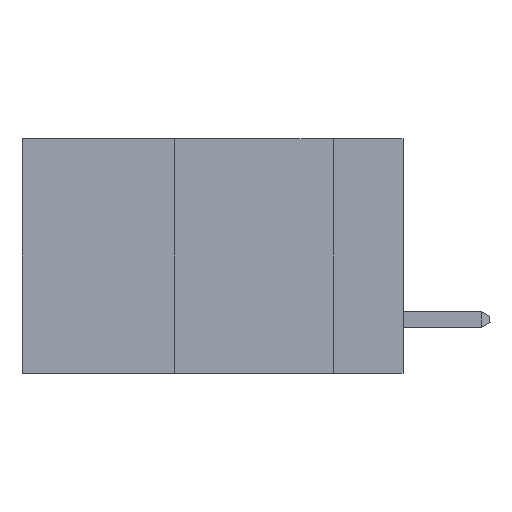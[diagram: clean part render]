
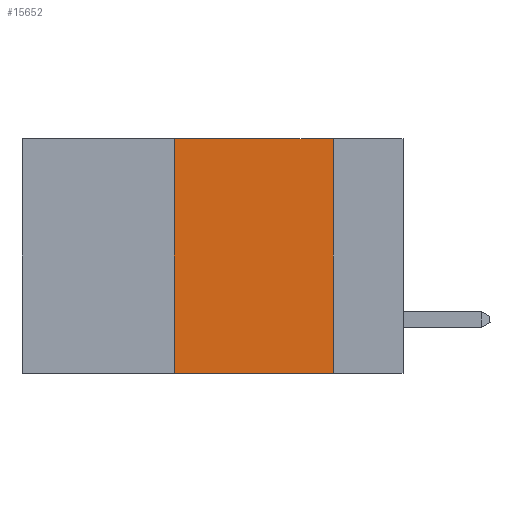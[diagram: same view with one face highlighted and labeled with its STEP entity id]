
A CAD part, left-side view. The second image highlights one B-rep face of the part: STEP entity #15652.
In plain terms, the highlighted planar face has unit normal (-1, 0, 0).
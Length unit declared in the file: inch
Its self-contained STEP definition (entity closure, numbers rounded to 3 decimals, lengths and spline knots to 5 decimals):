
#562 = LINE ( 'NONE', #15142, #16602 ) ;
#1436 = ORIENTED_EDGE ( 'NONE', *, *, #16681, .F. ) ;
#2051 = ORIENTED_EDGE ( 'NONE', *, *, #22466, .F. ) ;
#2705 = AXIS2_PLACEMENT_3D ( 'NONE', #6401, #4744, #6959 ) ;
#2799 = VERTEX_POINT ( 'NONE', #17373 ) ;
#4117 = DIRECTION ( 'NONE',  ( 0., 0., -1. ) ) ;
#4744 = DIRECTION ( 'NONE',  ( 1., 0., 0. ) ) ;
#5001 = VERTEX_POINT ( 'NONE', #19308 ) ;
#5289 = EDGE_CURVE ( 'NONE', #13646, #2799, #16895, .T. ) ;
#5386 = VECTOR ( 'NONE', #22765, 39.37008 ) ;
#6401 = CARTESIAN_POINT ( 'NONE',  ( 0., 0.6, 0. ) ) ;
#6959 = DIRECTION ( 'NONE',  ( 0., 0., -1. ) ) ;
#7456 = VECTOR ( 'NONE', #4117, 39.37008 ) ;
#7738 = VECTOR ( 'NONE', #8998, 39.37008 ) ;
#8998 = DIRECTION ( 'NONE',  ( 0., -1., 0. ) ) ;
#10690 = ORIENTED_EDGE ( 'NONE', *, *, #5289, .F. ) ;
#10766 = CARTESIAN_POINT ( 'NONE',  ( 0., 0.6, -0.37 ) ) ;
#10952 = VERTEX_POINT ( 'NONE', #13691 ) ;
#11803 = CARTESIAN_POINT ( 'NONE',  ( 0., 0.6, 0. ) ) ;
#13646 = VERTEX_POINT ( 'NONE', #13832 ) ;
#13691 = CARTESIAN_POINT ( 'NONE',  ( 0., 0.11, -0.37 ) ) ;
#13832 = CARTESIAN_POINT ( 'NONE',  ( 0., 0.36, 0. ) ) ;
#14056 = EDGE_LOOP ( 'NONE', ( #2051, #10690, #1436, #18895 ) ) ;
#15142 = CARTESIAN_POINT ( 'NONE',  ( 0., 0.36, 0. ) ) ;
#15652 = ADVANCED_FACE ( 'NONE', ( #22976 ), #20974, .F. ) ;
#16514 = EDGE_CURVE ( 'NONE', #5001, #10952, #16894, .T. ) ;
#16602 = VECTOR ( 'NONE', #20657, 39.37008 ) ;
#16613 = LINE ( 'NONE', #22393, #7456 ) ;
#16681 = EDGE_CURVE ( 'NONE', #5001, #13646, #562, .T. ) ;
#16894 = LINE ( 'NONE', #10766, #7738 ) ;
#16895 = LINE ( 'NONE', #11803, #5386 ) ;
#17373 = CARTESIAN_POINT ( 'NONE',  ( 0., 0.11, 0. ) ) ;
#18895 = ORIENTED_EDGE ( 'NONE', *, *, #16514, .T. ) ;
#19308 = CARTESIAN_POINT ( 'NONE',  ( 0., 0.36, -0.37 ) ) ;
#20657 = DIRECTION ( 'NONE',  ( 0., 0., 1. ) ) ;
#20974 = PLANE ( 'NONE',  #2705 ) ;
#22393 = CARTESIAN_POINT ( 'NONE',  ( 0., 0.11, 0. ) ) ;
#22466 = EDGE_CURVE ( 'NONE', #2799, #10952, #16613, .T. ) ;
#22765 = DIRECTION ( 'NONE',  ( 0., -1., 0. ) ) ;
#22976 = FACE_OUTER_BOUND ( 'NONE', #14056, .T. ) ;
